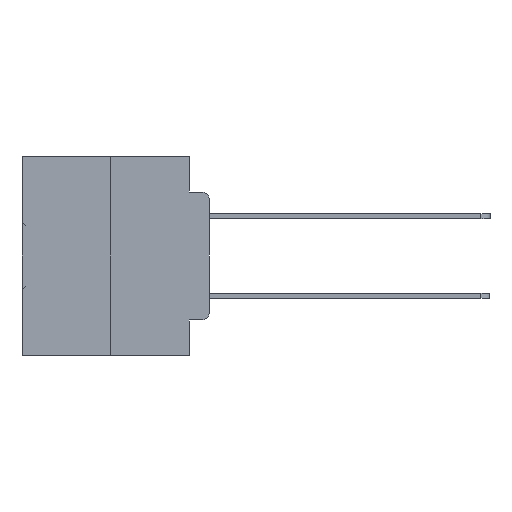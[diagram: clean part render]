
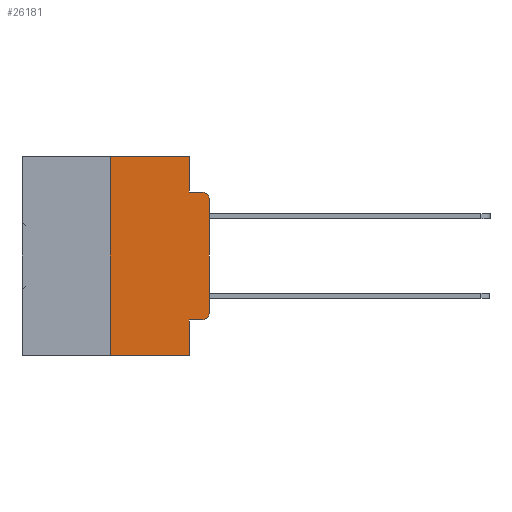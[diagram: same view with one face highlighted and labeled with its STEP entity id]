
A CAD part, left-side view. The second image highlights one B-rep face of the part: STEP entity #26181.
In plain terms, the highlighted planar face has unit normal (-1, 0, 0).
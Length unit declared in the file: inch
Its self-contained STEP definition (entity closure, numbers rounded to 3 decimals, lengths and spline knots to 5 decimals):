
#72 = ORIENTED_EDGE ( 'NONE', *, *, #30535, .F. ) ;
#487 = DIRECTION ( 'NONE',  ( 0., 0., -1. ) ) ;
#985 = VERTEX_POINT ( 'NONE', #11269 ) ;
#1395 = ORIENTED_EDGE ( 'NONE', *, *, #3561, .T. ) ;
#1498 = VERTEX_POINT ( 'NONE', #17760 ) ;
#1580 = ORIENTED_EDGE ( 'NONE', *, *, #25272, .T. ) ;
#2179 = FACE_OUTER_BOUND ( 'NONE', #6595, .T. ) ;
#2351 = DIRECTION ( 'NONE',  ( 0., 0., -1. ) ) ;
#3561 = EDGE_CURVE ( 'NONE', #29309, #985, #30879, .T. ) ;
#3919 = LINE ( 'NONE', #13601, #30759 ) ;
#4336 = CARTESIAN_POINT ( 'NONE',  ( 0., 0., 0. ) ) ;
#4494 = DIRECTION ( 'NONE',  ( -1., 0., 0. ) ) ;
#4500 = DIRECTION ( 'NONE',  ( 0., 0., -1. ) ) ;
#4692 = EDGE_CURVE ( 'NONE', #985, #29084, #28292, .T. ) ;
#4719 = CARTESIAN_POINT ( 'NONE',  ( 0., 0.02, -0.3915 ) ) ;
#6028 = CARTESIAN_POINT ( 'NONE',  ( 0., 0.25, -0.5 ) ) ;
#6595 = EDGE_LOOP ( 'NONE', ( #1580, #32351, #72, #21715, #9013, #17899, #33599, #14954, #1395, #30810 ) ) ;
#6699 = DIRECTION ( 'NONE',  ( 0., -1., 0. ) ) ;
#8042 = DIRECTION ( 'NONE',  ( 0., 0., -1. ) ) ;
#8063 = EDGE_CURVE ( 'NONE', #26924, #20160, #32508, .T. ) ;
#9013 = ORIENTED_EDGE ( 'NONE', *, *, #22530, .F. ) ;
#10418 = CARTESIAN_POINT ( 'NONE',  ( 0., 0.473, 0. ) ) ;
#10809 = CARTESIAN_POINT ( 'NONE',  ( 0., 0.051, 0. ) ) ;
#11269 = CARTESIAN_POINT ( 'NONE',  ( 0., 0.02, -0.4115 ) ) ;
#12051 = VERTEX_POINT ( 'NONE', #16763 ) ;
#12242 = LINE ( 'NONE', #23838, #32596 ) ;
#12247 = AXIS2_PLACEMENT_3D ( 'NONE', #32558, #16698, #487 ) ;
#13078 = LINE ( 'NONE', #24790, #33425 ) ;
#13601 = CARTESIAN_POINT ( 'NONE',  ( 0., 0.051, 0. ) ) ;
#14629 = CARTESIAN_POINT ( 'NONE',  ( 0., 0.051, -0.0885 ) ) ;
#14954 = ORIENTED_EDGE ( 'NONE', *, *, #19876, .F. ) ;
#15079 = CARTESIAN_POINT ( 'NONE',  ( 0., 0.25, 0. ) ) ;
#15856 = PLANE ( 'NONE',  #32593 ) ;
#16425 = CARTESIAN_POINT ( 'NONE',  ( 0., 0.02, -0.0885 ) ) ;
#16698 = DIRECTION ( 'NONE',  ( -1., 0., 0. ) ) ;
#16763 = CARTESIAN_POINT ( 'NONE',  ( 0., 0., -0.1085 ) ) ;
#17328 = AXIS2_PLACEMENT_3D ( 'NONE', #4719, #4494, #4500 ) ;
#17398 = CARTESIAN_POINT ( 'NONE',  ( 0., 0.051, -0.5 ) ) ;
#17733 = VECTOR ( 'NONE', #22529, 39.37008 ) ;
#17760 = CARTESIAN_POINT ( 'NONE',  ( 0., 0.051, 0. ) ) ;
#17899 = ORIENTED_EDGE ( 'NONE', *, *, #27653, .F. ) ;
#18376 = DIRECTION ( 'NONE',  ( 0., -1., 0. ) ) ;
#18401 = DIRECTION ( 'NONE',  ( 0., -1., 0. ) ) ;
#18446 = VECTOR ( 'NONE', #18376, 39.37008 ) ;
#18564 = DIRECTION ( 'NONE',  ( 1., 0., 0. ) ) ;
#19876 = EDGE_CURVE ( 'NONE', #29309, #20160, #30400, .T. ) ;
#20160 = VERTEX_POINT ( 'NONE', #17398 ) ;
#20531 = DIRECTION ( 'NONE',  ( 0., 0., 1. ) ) ;
#20552 = CARTESIAN_POINT ( 'NONE',  ( 0., 0., -0.3915 ) ) ;
#20560 = EDGE_CURVE ( 'NONE', #1498, #29012, #3919, .T. ) ;
#20574 = VERTEX_POINT ( 'NONE', #16425 ) ;
#21691 = DIRECTION ( 'NONE',  ( 0., 0., -1. ) ) ;
#21715 = ORIENTED_EDGE ( 'NONE', *, *, #20560, .F. ) ;
#22529 = DIRECTION ( 'NONE',  ( 0., 0., 1. ) ) ;
#22530 = EDGE_CURVE ( 'NONE', #31903, #1498, #13078, .T. ) ;
#23406 = VECTOR ( 'NONE', #21691, 39.37008 ) ;
#23838 = CARTESIAN_POINT ( 'NONE',  ( 0., 0.051, -0.0885 ) ) ;
#24671 = VECTOR ( 'NONE', #20531, 39.37008 ) ;
#24790 = CARTESIAN_POINT ( 'NONE',  ( 0., 0.473, 0. ) ) ;
#25192 = CARTESIAN_POINT ( 'NONE',  ( 0., 0.25, 0. ) ) ;
#25272 = EDGE_CURVE ( 'NONE', #29084, #12051, #25493, .T. ) ;
#25493 = LINE ( 'NONE', #4336, #24671 ) ;
#26181 = ADVANCED_FACE ( 'NONE', ( #2179 ), #15856, .F. ) ;
#26924 = VERTEX_POINT ( 'NONE', #6028 ) ;
#27402 = DIRECTION ( 'NONE',  ( 0., -1., 0. ) ) ;
#27653 = EDGE_CURVE ( 'NONE', #26924, #31903, #32627, .T. ) ;
#28292 = CIRCLE ( 'NONE', #17328, 0.02 ) ;
#28387 = CARTESIAN_POINT ( 'NONE',  ( 0., 0.051, -0.4115 ) ) ;
#29012 = VERTEX_POINT ( 'NONE', #14629 ) ;
#29084 = VERTEX_POINT ( 'NONE', #20552 ) ;
#29309 = VERTEX_POINT ( 'NONE', #34583 ) ;
#30052 = VECTOR ( 'NONE', #6699, 39.37008 ) ;
#30400 = LINE ( 'NONE', #10809, #23406 ) ;
#30535 = EDGE_CURVE ( 'NONE', #29012, #20574, #12242, .T. ) ;
#30759 = VECTOR ( 'NONE', #8042, 39.37008 ) ;
#30810 = ORIENTED_EDGE ( 'NONE', *, *, #4692, .T. ) ;
#30879 = LINE ( 'NONE', #28387, #30052 ) ;
#31590 = CARTESIAN_POINT ( 'NONE',  ( 0., 0.473, -0.5 ) ) ;
#31903 = VERTEX_POINT ( 'NONE', #15079 ) ;
#32230 = EDGE_CURVE ( 'NONE', #12051, #20574, #34513, .T. ) ;
#32351 = ORIENTED_EDGE ( 'NONE', *, *, #32230, .T. ) ;
#32508 = LINE ( 'NONE', #31590, #18446 ) ;
#32558 = CARTESIAN_POINT ( 'NONE',  ( 0., 0.02, -0.1085 ) ) ;
#32593 = AXIS2_PLACEMENT_3D ( 'NONE', #10418, #18564, #2351 ) ;
#32596 = VECTOR ( 'NONE', #18401, 39.37008 ) ;
#32627 = LINE ( 'NONE', #25192, #17733 ) ;
#33425 = VECTOR ( 'NONE', #27402, 39.37008 ) ;
#33599 = ORIENTED_EDGE ( 'NONE', *, *, #8063, .T. ) ;
#34513 = CIRCLE ( 'NONE', #12247, 0.02 ) ;
#34583 = CARTESIAN_POINT ( 'NONE',  ( 0., 0.051, -0.4115 ) ) ;
